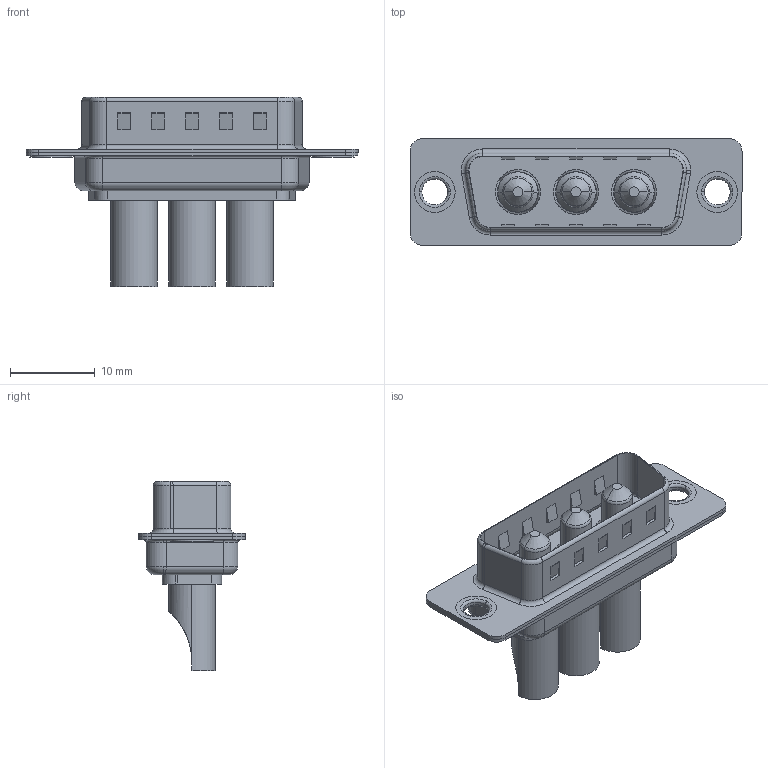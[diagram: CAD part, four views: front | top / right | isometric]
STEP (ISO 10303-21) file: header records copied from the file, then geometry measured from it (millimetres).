
FILE_DESCRIPTION (( 'STEP AP203' ), '1' );
FILE_NAME ('627-3W3-222-4N1.STEP', '2019-05-24T13:02:51', ( '' ), ( '' ), 'SwSTEP 2.0', 'SolidWorks 2016', '' );
FILE_SCHEMA (( 'CONFIG_CONTROL_DESIGN' ));
Length unit declared in the file: millimetre
Products named in the file (6): 627Combo Housing_3W3; 627Combo Shell Rear_15 Contacts; 627Combo Shell Front_15 Contacts; 627Combo Thru Hole Rivet; Power Pin_40A SC; 627-3W3-222-4N1
Assembly tree (8 placements, depth 2):
  627-3W3-222-4N1
    627Combo Housing_3W3
    627Combo Shell Rear_15 Contacts
    627Combo Shell Front_15 Contacts
    627Combo Thru Hole Rivet  x2
    Power Pin_40A SC  x3
Bounding box: 39.15 x 12.6 x 22.3 mm (x, y, z)
Volume: 2090.9 mm3; surface area: 4980.9 mm2
Topology: 11 solids, 11 shells, 443 faces, 1063 edges, 653 vertices
Faces by surface type: cylinder 177, plane 175, torus 64, cone 21, bspline 6
Entity records: 11132 total; most frequent: CARTESIAN_POINT 1921, DIRECTION 1887, ORIENTED_EDGE 1702, EDGE_CURVE 851, AXIS2_PLACEMENT_3D 703, VERTEX_POINT 531, LINE 481, VECTOR 481
